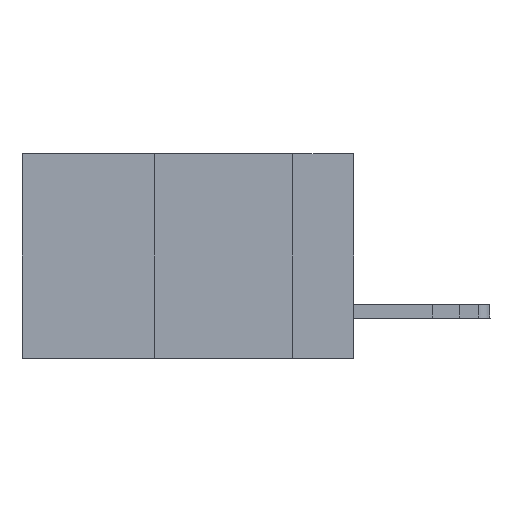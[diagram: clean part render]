
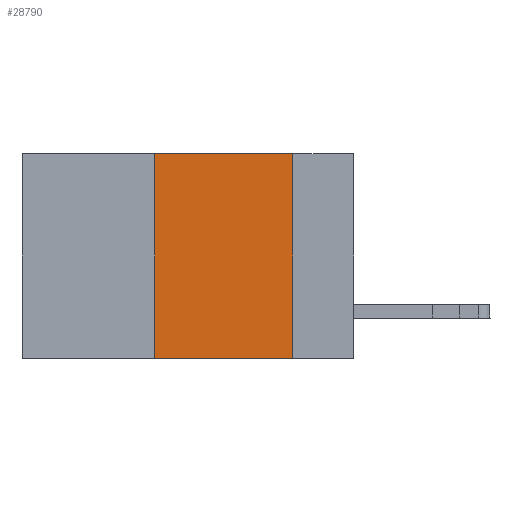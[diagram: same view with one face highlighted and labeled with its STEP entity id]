
A CAD part, left-side view. The second image highlights one B-rep face of the part: STEP entity #28790.
In plain terms, the highlighted planar face has unit normal (-1, 0, 0).
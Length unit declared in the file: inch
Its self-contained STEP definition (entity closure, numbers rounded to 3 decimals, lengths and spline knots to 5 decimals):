
#955 = AXIS2_PLACEMENT_3D ( 'NONE', #1783, #24940, #25529 ) ;
#1783 = CARTESIAN_POINT ( 'NONE',  ( 0., 0.6, 0. ) ) ;
#1797 = VERTEX_POINT ( 'NONE', #2945 ) ;
#1799 = CARTESIAN_POINT ( 'NONE',  ( 0., 0.6, 0. ) ) ;
#2945 = CARTESIAN_POINT ( 'NONE',  ( 0., 0.11, -0.37 ) ) ;
#3467 = CARTESIAN_POINT ( 'NONE',  ( 0., 0.11, 0. ) ) ;
#4996 = EDGE_CURVE ( 'NONE', #34526, #27833, #8001, .T. ) ;
#5780 = VECTOR ( 'NONE', #27904, 39.37008 ) ;
#8001 = LINE ( 'NONE', #1799, #5780 ) ;
#9451 = CARTESIAN_POINT ( 'NONE',  ( 0., 0.36, 0. ) ) ;
#9700 = DIRECTION ( 'NONE',  ( 0., -1., 0. ) ) ;
#10342 = PLANE ( 'NONE',  #955 ) ;
#10874 = EDGE_LOOP ( 'NONE', ( #35202, #26361, #21451, #30801 ) ) ;
#12633 = CARTESIAN_POINT ( 'NONE',  ( 0., 0.6, -0.37 ) ) ;
#16215 = FACE_OUTER_BOUND ( 'NONE', #10874, .T. ) ;
#16750 = CARTESIAN_POINT ( 'NONE',  ( 0., 0.36, -0.37 ) ) ;
#17594 = EDGE_CURVE ( 'NONE', #30696, #1797, #36791, .T. ) ;
#21451 = ORIENTED_EDGE ( 'NONE', *, *, #29480, .F. ) ;
#24940 = DIRECTION ( 'NONE',  ( 1., 0., 0. ) ) ;
#25529 = DIRECTION ( 'NONE',  ( 0., 0., -1. ) ) ;
#26210 = LINE ( 'NONE', #32264, #26533 ) ;
#26361 = ORIENTED_EDGE ( 'NONE', *, *, #4996, .F. ) ;
#26533 = VECTOR ( 'NONE', #34789, 39.37008 ) ;
#27190 = LINE ( 'NONE', #9451, #29030 ) ;
#27833 = VERTEX_POINT ( 'NONE', #3467 ) ;
#27904 = DIRECTION ( 'NONE',  ( 0., -1., 0. ) ) ;
#28790 = ADVANCED_FACE ( 'NONE', ( #16215 ), #10342, .F. ) ;
#29030 = VECTOR ( 'NONE', #32673, 39.37008 ) ;
#29480 = EDGE_CURVE ( 'NONE', #30696, #34526, #27190, .T. ) ;
#29764 = EDGE_CURVE ( 'NONE', #27833, #1797, #26210, .T. ) ;
#30481 = VECTOR ( 'NONE', #9700, 39.37008 ) ;
#30696 = VERTEX_POINT ( 'NONE', #16750 ) ;
#30801 = ORIENTED_EDGE ( 'NONE', *, *, #17594, .T. ) ;
#32264 = CARTESIAN_POINT ( 'NONE',  ( 0., 0.11, 0. ) ) ;
#32673 = DIRECTION ( 'NONE',  ( 0., 0., 1. ) ) ;
#34526 = VERTEX_POINT ( 'NONE', #36861 ) ;
#34789 = DIRECTION ( 'NONE',  ( 0., 0., -1. ) ) ;
#35202 = ORIENTED_EDGE ( 'NONE', *, *, #29764, .F. ) ;
#36791 = LINE ( 'NONE', #12633, #30481 ) ;
#36861 = CARTESIAN_POINT ( 'NONE',  ( 0., 0.36, 0. ) ) ;
